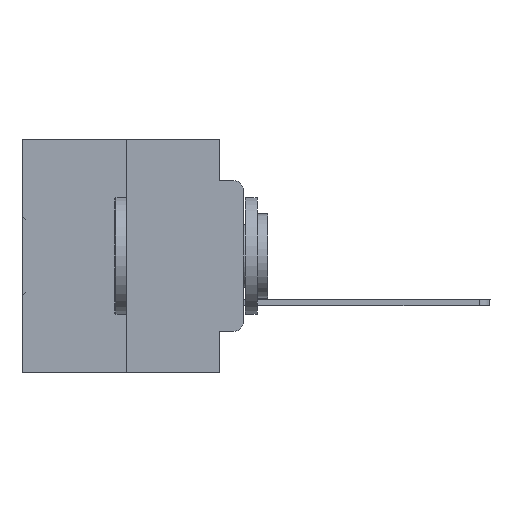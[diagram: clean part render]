
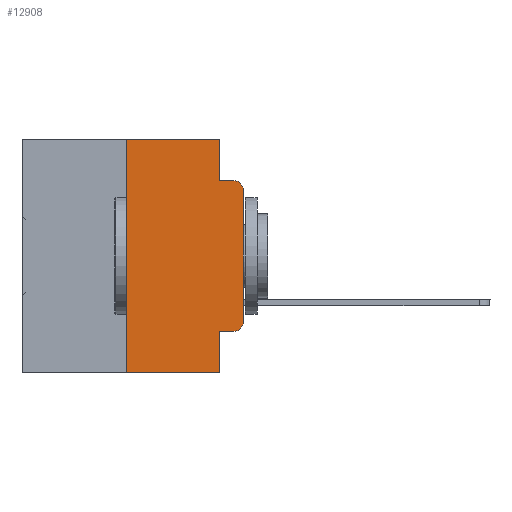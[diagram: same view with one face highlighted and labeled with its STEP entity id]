
A CAD part, left-side view. The second image highlights one B-rep face of the part: STEP entity #12908.
In plain terms, the highlighted planar face has unit normal (-1, 0, 0).
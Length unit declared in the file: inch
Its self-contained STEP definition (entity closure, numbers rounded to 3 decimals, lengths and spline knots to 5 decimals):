
#270 = VERTEX_POINT ( 'NONE', #33303 ) ;
#306 = ORIENTED_EDGE ( 'NONE', *, *, #9753, .F. ) ;
#537 = CARTESIAN_POINT ( 'NONE',  ( 0., 0.02, -0.3915 ) ) ;
#544 = EDGE_CURVE ( 'NONE', #23978, #15251, #13161, .T. ) ;
#1358 = DIRECTION ( 'NONE',  ( 0., -1., 0. ) ) ;
#1694 = FACE_OUTER_BOUND ( 'NONE', #21247, .T. ) ;
#1883 = DIRECTION ( 'NONE',  ( 1., 0., 0. ) ) ;
#2695 = VECTOR ( 'NONE', #21093, 39.37008 ) ;
#2974 = CARTESIAN_POINT ( 'NONE',  ( 0., 0.051, 0. ) ) ;
#3506 = DIRECTION ( 'NONE',  ( 0., 0., 1. ) ) ;
#3615 = DIRECTION ( 'NONE',  ( 0., 0., -1. ) ) ;
#3696 = CARTESIAN_POINT ( 'NONE',  ( 0., 0.051, 0. ) ) ;
#3856 = EDGE_CURVE ( 'NONE', #21809, #25727, #10765, .T. ) ;
#4038 = CARTESIAN_POINT ( 'NONE',  ( 0., 0.02, -0.1085 ) ) ;
#4671 = VERTEX_POINT ( 'NONE', #10841 ) ;
#4867 = EDGE_CURVE ( 'NONE', #4671, #7843, #21445, .T. ) ;
#6711 = DIRECTION ( 'NONE',  ( 0., 0., 1. ) ) ;
#6713 = EDGE_CURVE ( 'NONE', #7843, #19518, #12488, .T. ) ;
#6792 = VERTEX_POINT ( 'NONE', #31720 ) ;
#6885 = CARTESIAN_POINT ( 'NONE',  ( 0., 0., 0. ) ) ;
#7130 = ORIENTED_EDGE ( 'NONE', *, *, #544, .F. ) ;
#7237 = VERTEX_POINT ( 'NONE', #9198 ) ;
#7534 = ORIENTED_EDGE ( 'NONE', *, *, #34980, .T. ) ;
#7541 = VECTOR ( 'NONE', #33041, 39.37008 ) ;
#7843 = VERTEX_POINT ( 'NONE', #10409 ) ;
#8213 = LINE ( 'NONE', #2974, #22806 ) ;
#8296 = VECTOR ( 'NONE', #1358, 39.37008 ) ;
#8305 = ORIENTED_EDGE ( 'NONE', *, *, #6713, .T. ) ;
#8931 = DIRECTION ( 'NONE',  ( 0., 0., -1. ) ) ;
#9198 = CARTESIAN_POINT ( 'NONE',  ( 0., 0.051, -0.4115 ) ) ;
#9300 = CARTESIAN_POINT ( 'NONE',  ( 0., 0.473, -0.5 ) ) ;
#9595 = EDGE_CURVE ( 'NONE', #15251, #21809, #8213, .T. ) ;
#9724 = CARTESIAN_POINT ( 'NONE',  ( 0., 0.02, -0.0885 ) ) ;
#9753 = EDGE_CURVE ( 'NONE', #270, #23978, #19737, .T. ) ;
#10331 = ORIENTED_EDGE ( 'NONE', *, *, #3856, .F. ) ;
#10409 = CARTESIAN_POINT ( 'NONE',  ( 0., 0., -0.3915 ) ) ;
#10765 = LINE ( 'NONE', #16713, #12635 ) ;
#10841 = CARTESIAN_POINT ( 'NONE',  ( 0., 0.02, -0.4115 ) ) ;
#12488 = LINE ( 'NONE', #6885, #13230 ) ;
#12635 = VECTOR ( 'NONE', #30352, 39.37008 ) ;
#12908 = ADVANCED_FACE ( 'NONE', ( #1694 ), #24027, .F. ) ;
#13161 = LINE ( 'NONE', #21446, #2695 ) ;
#13230 = VECTOR ( 'NONE', #6711, 39.37008 ) ;
#13471 = CARTESIAN_POINT ( 'NONE',  ( 0., 0.051, -0.4115 ) ) ;
#13985 = DIRECTION ( 'NONE',  ( 0., 0., -1. ) ) ;
#15016 = ORIENTED_EDGE ( 'NONE', *, *, #15614, .F. ) ;
#15251 = VERTEX_POINT ( 'NONE', #23530 ) ;
#15614 = EDGE_CURVE ( 'NONE', #7237, #6792, #22614, .T. ) ;
#16713 = CARTESIAN_POINT ( 'NONE',  ( 0., 0.051, -0.0885 ) ) ;
#16733 = EDGE_CURVE ( 'NONE', #7237, #4671, #19047, .T. ) ;
#17317 = DIRECTION ( 'NONE',  ( -1., 0., 0. ) ) ;
#17772 = AXIS2_PLACEMENT_3D ( 'NONE', #18118, #1883, #20812 ) ;
#17915 = DIRECTION ( 'NONE',  ( 0., 0., -1. ) ) ;
#18118 = CARTESIAN_POINT ( 'NONE',  ( 0., 0.473, 0. ) ) ;
#19000 = CARTESIAN_POINT ( 'NONE',  ( 0., 0.25, 0. ) ) ;
#19047 = LINE ( 'NONE', #13471, #7541 ) ;
#19162 = CARTESIAN_POINT ( 'NONE',  ( 0., 0., -0.1085 ) ) ;
#19518 = VERTEX_POINT ( 'NONE', #19162 ) ;
#19737 = LINE ( 'NONE', #31378, #20376 ) ;
#20376 = VECTOR ( 'NONE', #3506, 39.37008 ) ;
#20812 = DIRECTION ( 'NONE',  ( 0., 0., -1. ) ) ;
#21015 = ORIENTED_EDGE ( 'NONE', *, *, #31970, .T. ) ;
#21093 = DIRECTION ( 'NONE',  ( 0., -1., 0. ) ) ;
#21247 = EDGE_LOOP ( 'NONE', ( #8305, #7534, #10331, #29065, #7130, #306, #21015, #15016, #33713, #26678 ) ) ;
#21445 = CIRCLE ( 'NONE', #25464, 0.02 ) ;
#21446 = CARTESIAN_POINT ( 'NONE',  ( 0., 0.473, 0. ) ) ;
#21809 = VERTEX_POINT ( 'NONE', #22830 ) ;
#22614 = LINE ( 'NONE', #3696, #33871 ) ;
#22806 = VECTOR ( 'NONE', #13985, 39.37008 ) ;
#22830 = CARTESIAN_POINT ( 'NONE',  ( 0., 0.051, -0.0885 ) ) ;
#23530 = CARTESIAN_POINT ( 'NONE',  ( 0., 0.051, 0. ) ) ;
#23978 = VERTEX_POINT ( 'NONE', #19000 ) ;
#24027 = PLANE ( 'NONE',  #17772 ) ;
#25464 = AXIS2_PLACEMENT_3D ( 'NONE', #537, #17317, #3615 ) ;
#25727 = VERTEX_POINT ( 'NONE', #9724 ) ;
#26678 = ORIENTED_EDGE ( 'NONE', *, *, #4867, .T. ) ;
#28496 = DIRECTION ( 'NONE',  ( -1., 0., 0. ) ) ;
#29065 = ORIENTED_EDGE ( 'NONE', *, *, #9595, .F. ) ;
#30352 = DIRECTION ( 'NONE',  ( 0., -1., 0. ) ) ;
#31378 = CARTESIAN_POINT ( 'NONE',  ( 0., 0.25, 0. ) ) ;
#31720 = CARTESIAN_POINT ( 'NONE',  ( 0., 0.051, -0.5 ) ) ;
#31970 = EDGE_CURVE ( 'NONE', #270, #6792, #34294, .T. ) ;
#33041 = DIRECTION ( 'NONE',  ( 0., -1., 0. ) ) ;
#33303 = CARTESIAN_POINT ( 'NONE',  ( 0., 0.25, -0.5 ) ) ;
#33713 = ORIENTED_EDGE ( 'NONE', *, *, #16733, .T. ) ;
#33871 = VECTOR ( 'NONE', #8931, 39.37008 ) ;
#34294 = LINE ( 'NONE', #9300, #8296 ) ;
#34563 = CIRCLE ( 'NONE', #35165, 0.02 ) ;
#34980 = EDGE_CURVE ( 'NONE', #19518, #25727, #34563, .T. ) ;
#35165 = AXIS2_PLACEMENT_3D ( 'NONE', #4038, #28496, #17915 ) ;
